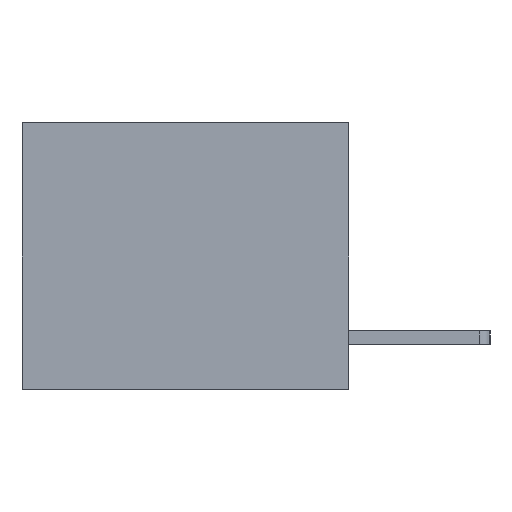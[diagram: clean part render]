
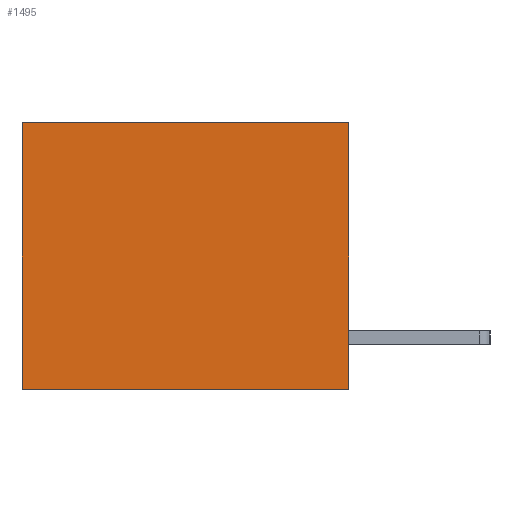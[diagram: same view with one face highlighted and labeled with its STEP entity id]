
A CAD part, left-side view. The second image highlights one B-rep face of the part: STEP entity #1495.
In plain terms, the highlighted planar face has unit normal (-1, 0, 0).
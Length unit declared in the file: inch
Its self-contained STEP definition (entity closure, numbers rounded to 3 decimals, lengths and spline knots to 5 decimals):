
#59 = CARTESIAN_POINT ( 'NONE',  ( 0.3165, 0.6, -0.49 ) ) ;
#479 = ORIENTED_EDGE ( 'NONE', *, *, #13600, .T. ) ;
#528 = LINE ( 'NONE', #3637, #4447 ) ;
#788 = VERTEX_POINT ( 'NONE', #4208 ) ;
#841 = CARTESIAN_POINT ( 'NONE',  ( 0.3165, 0., -0.49 ) ) ;
#905 = CARTESIAN_POINT ( 'NONE',  ( 0.3165, 0., 0. ) ) ;
#1495 = ADVANCED_FACE ( 'NONE', ( #9802 ), #4123, .F. ) ;
#1779 = VERTEX_POINT ( 'NONE', #6448 ) ;
#2262 = DIRECTION ( 'NONE',  ( 0., 0., -1. ) ) ;
#2281 = VERTEX_POINT ( 'NONE', #7285 ) ;
#2676 = EDGE_CURVE ( 'NONE', #788, #5027, #528, .T. ) ;
#3089 = CARTESIAN_POINT ( 'NONE',  ( 0.3165, 0., -0.49 ) ) ;
#3280 = AXIS2_PLACEMENT_3D ( 'NONE', #841, #12891, #5231 ) ;
#3349 = EDGE_CURVE ( 'NONE', #1779, #788, #3925, .T. ) ;
#3637 = CARTESIAN_POINT ( 'NONE',  ( 0.3165, 0., -0.49 ) ) ;
#3925 = LINE ( 'NONE', #3089, #12355 ) ;
#4123 = PLANE ( 'NONE',  #3280 ) ;
#4208 = CARTESIAN_POINT ( 'NONE',  ( 0.3165, 0., -0.49 ) ) ;
#4447 = VECTOR ( 'NONE', #10052, 39.37008 ) ;
#4493 = CARTESIAN_POINT ( 'NONE',  ( 0.3165, 0.6, -0.49 ) ) ;
#4728 = VECTOR ( 'NONE', #11852, 39.37008 ) ;
#5027 = VERTEX_POINT ( 'NONE', #4493 ) ;
#5231 = DIRECTION ( 'NONE',  ( 0., 0., -1. ) ) ;
#5600 = LINE ( 'NONE', #905, #4728 ) ;
#6448 = CARTESIAN_POINT ( 'NONE',  ( 0.3165, 0., 0. ) ) ;
#7212 = EDGE_CURVE ( 'NONE', #1779, #2281, #5600, .T. ) ;
#7285 = CARTESIAN_POINT ( 'NONE',  ( 0.3165, 0.6, 0. ) ) ;
#7322 = ORIENTED_EDGE ( 'NONE', *, *, #2676, .F. ) ;
#7344 = ORIENTED_EDGE ( 'NONE', *, *, #7212, .T. ) ;
#7728 = VECTOR ( 'NONE', #2262, 39.37008 ) ;
#9802 = FACE_OUTER_BOUND ( 'NONE', #14094, .T. ) ;
#10052 = DIRECTION ( 'NONE',  ( 0., 1., 0. ) ) ;
#11726 = ORIENTED_EDGE ( 'NONE', *, *, #3349, .F. ) ;
#11852 = DIRECTION ( 'NONE',  ( 0., 1., 0. ) ) ;
#12355 = VECTOR ( 'NONE', #12816, 39.37008 ) ;
#12816 = DIRECTION ( 'NONE',  ( 0., 0., -1. ) ) ;
#12891 = DIRECTION ( 'NONE',  ( 1., 0., 0. ) ) ;
#13446 = LINE ( 'NONE', #59, #7728 ) ;
#13600 = EDGE_CURVE ( 'NONE', #2281, #5027, #13446, .T. ) ;
#14094 = EDGE_LOOP ( 'NONE', ( #479, #7322, #11726, #7344 ) ) ;
